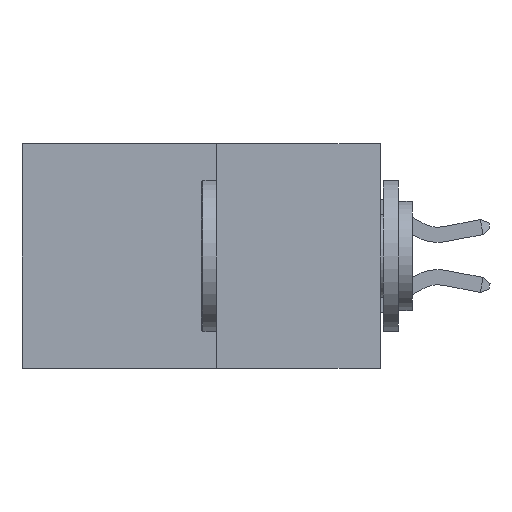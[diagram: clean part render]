
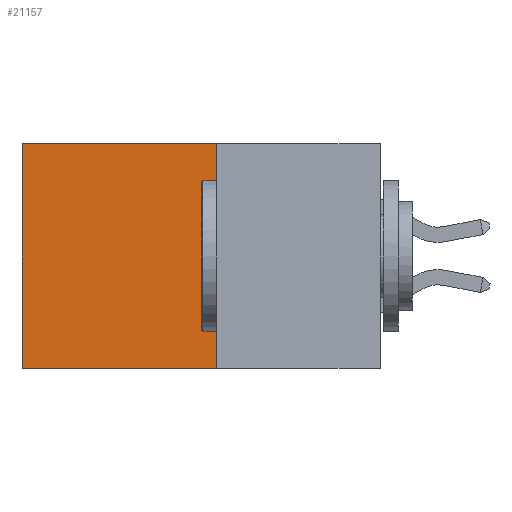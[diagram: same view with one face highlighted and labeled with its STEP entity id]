
A CAD part, left-side view. The second image highlights one B-rep face of the part: STEP entity #21157.
In plain terms, the highlighted planar face has unit normal (-1, 0, 0).
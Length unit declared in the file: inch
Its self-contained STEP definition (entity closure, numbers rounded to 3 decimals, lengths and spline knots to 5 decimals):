
#194 = ORIENTED_EDGE ( 'NONE', *, *, #21433, .T. ) ;
#1185 = EDGE_CURVE ( 'NONE', #8589, #14112, #8006, .T. ) ;
#1942 = DIRECTION ( 'NONE',  ( 0., 0., -1. ) ) ;
#2144 = DIRECTION ( 'NONE',  ( 1., 0., 0. ) ) ;
#2615 = VECTOR ( 'NONE', #23149, 39.37008 ) ;
#2940 = CARTESIAN_POINT ( 'NONE',  ( 0.277, 0.59, -0.37 ) ) ;
#3844 = CARTESIAN_POINT ( 'NONE',  ( 0.277, 0.27, -0.37 ) ) ;
#4790 = DIRECTION ( 'NONE',  ( 0., 1., 0. ) ) ;
#5879 = CARTESIAN_POINT ( 'NONE',  ( 0.277, 0.27, -0.37 ) ) ;
#6121 = AXIS2_PLACEMENT_3D ( 'NONE', #14227, #2144, #16199 ) ;
#6384 = EDGE_CURVE ( 'NONE', #9104, #22308, #7823, .T. ) ;
#7823 = LINE ( 'NONE', #3844, #23041 ) ;
#8006 = LINE ( 'NONE', #23474, #2615 ) ;
#8192 = PLANE ( 'NONE',  #6121 ) ;
#8589 = VERTEX_POINT ( 'NONE', #9960 ) ;
#9104 = VERTEX_POINT ( 'NONE', #9423 ) ;
#9423 = CARTESIAN_POINT ( 'NONE',  ( 0.277, 0.27, -0.37 ) ) ;
#9546 = CARTESIAN_POINT ( 'NONE',  ( 0.277, 0.59, -0.37 ) ) ;
#9960 = CARTESIAN_POINT ( 'NONE',  ( 0.277, 0.27, 0. ) ) ;
#10067 = ORIENTED_EDGE ( 'NONE', *, *, #1185, .T. ) ;
#11016 = ORIENTED_EDGE ( 'NONE', *, *, #6384, .F. ) ;
#11218 = EDGE_CURVE ( 'NONE', #8589, #9104, #23083, .T. ) ;
#13393 = CARTESIAN_POINT ( 'NONE',  ( 0.277, 0.59, 0. ) ) ;
#14112 = VERTEX_POINT ( 'NONE', #13393 ) ;
#14192 = LINE ( 'NONE', #2940, #14820 ) ;
#14227 = CARTESIAN_POINT ( 'NONE',  ( 0.277, 0.27, -0.37 ) ) ;
#14820 = VECTOR ( 'NONE', #16965, 39.37008 ) ;
#16199 = DIRECTION ( 'NONE',  ( 0., 0., -1. ) ) ;
#16206 = EDGE_LOOP ( 'NONE', ( #194, #11016, #21244, #10067 ) ) ;
#16965 = DIRECTION ( 'NONE',  ( 0., 0., -1. ) ) ;
#17819 = VECTOR ( 'NONE', #1942, 39.37008 ) ;
#19755 = FACE_OUTER_BOUND ( 'NONE', #16206, .T. ) ;
#21157 = ADVANCED_FACE ( 'NONE', ( #19755 ), #8192, .F. ) ;
#21244 = ORIENTED_EDGE ( 'NONE', *, *, #11218, .F. ) ;
#21433 = EDGE_CURVE ( 'NONE', #14112, #22308, #14192, .T. ) ;
#22308 = VERTEX_POINT ( 'NONE', #9546 ) ;
#23041 = VECTOR ( 'NONE', #4790, 39.37008 ) ;
#23083 = LINE ( 'NONE', #5879, #17819 ) ;
#23149 = DIRECTION ( 'NONE',  ( 0., 1., 0. ) ) ;
#23474 = CARTESIAN_POINT ( 'NONE',  ( 0.277, 0.27, 0. ) ) ;
